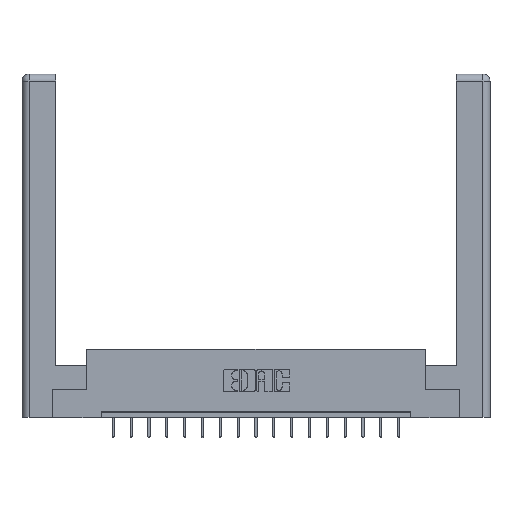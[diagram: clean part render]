
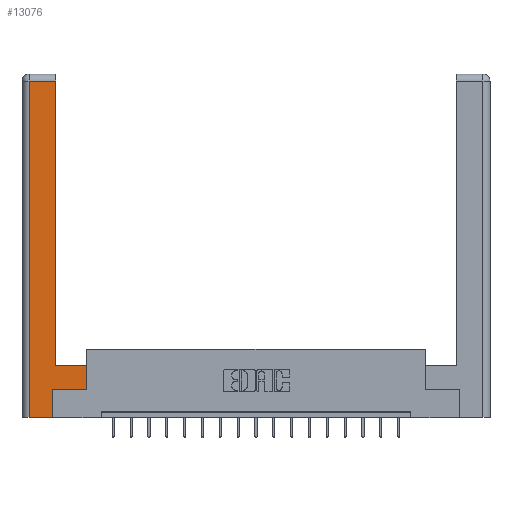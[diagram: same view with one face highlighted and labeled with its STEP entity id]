
A CAD part, top view. The second image highlights one B-rep face of the part: STEP entity #13076.
In plain terms, the highlighted planar face has unit normal (0, 0, 1).
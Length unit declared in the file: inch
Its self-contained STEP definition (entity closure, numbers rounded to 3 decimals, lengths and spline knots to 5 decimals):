
#678 = LINE ( 'NONE', #3868, #5820 ) ;
#895 = VERTEX_POINT ( 'NONE', #13260 ) ;
#1141 = CARTESIAN_POINT ( 'NONE',  ( 0.265, 0.245, 0. ) ) ;
#1548 = VERTEX_POINT ( 'NONE', #1141 ) ;
#2025 = CARTESIAN_POINT ( 'NONE',  ( 0.295, 3., 0. ) ) ;
#2036 = EDGE_CURVE ( 'NONE', #6035, #15443, #678, .T. ) ;
#2357 = DIRECTION ( 'NONE',  ( -1., 0., 0. ) ) ;
#2650 = VECTOR ( 'NONE', #15157, 39.37008 ) ;
#2853 = EDGE_CURVE ( 'NONE', #15443, #895, #17917, .T. ) ;
#3011 = DIRECTION ( 'NONE',  ( 0., 1., 0. ) ) ;
#3128 = DIRECTION ( 'NONE',  ( 1., 0., 0. ) ) ;
#3141 = VECTOR ( 'NONE', #3011, 39.37008 ) ;
#3716 = CARTESIAN_POINT ( 'NONE',  ( 0.265, 0.245, 0. ) ) ;
#3868 = CARTESIAN_POINT ( 'NONE',  ( 0.0615, 2.94, 0. ) ) ;
#4057 = LINE ( 'NONE', #2025, #3141 ) ;
#4668 = ORIENTED_EDGE ( 'NONE', *, *, #13338, .T. ) ;
#5416 = ORIENTED_EDGE ( 'NONE', *, *, #16015, .T. ) ;
#5820 = VECTOR ( 'NONE', #16786, 39.37008 ) ;
#5849 = VERTEX_POINT ( 'NONE', #10890 ) ;
#5963 = CARTESIAN_POINT ( 'NONE',  ( 0.265, 0., 0. ) ) ;
#6035 = VERTEX_POINT ( 'NONE', #12822 ) ;
#6521 = CARTESIAN_POINT ( 'NONE',  ( 0.0615, 0., 0. ) ) ;
#6703 = ORIENTED_EDGE ( 'NONE', *, *, #2036, .T. ) ;
#7491 = EDGE_CURVE ( 'NONE', #5849, #16542, #15803, .T. ) ;
#8021 = CARTESIAN_POINT ( 'NONE',  ( 0.0615, 2.94, 0. ) ) ;
#8182 = CARTESIAN_POINT ( 'NONE',  ( 0.565, 0.245, 0. ) ) ;
#8276 = CARTESIAN_POINT ( 'NONE',  ( 0.295, 0.45, 0. ) ) ;
#8299 = DIRECTION ( 'NONE',  ( 0., 0., -1. ) ) ;
#8716 = EDGE_CURVE ( 'NONE', #15977, #5849, #11734, .T. ) ;
#9403 = ORIENTED_EDGE ( 'NONE', *, *, #10560, .T. ) ;
#9497 = FACE_OUTER_BOUND ( 'NONE', #17702, .T. ) ;
#10161 = LINE ( 'NONE', #8182, #17144 ) ;
#10192 = AXIS2_PLACEMENT_3D ( 'NONE', #16948, #8299, #12683 ) ;
#10560 = EDGE_CURVE ( 'NONE', #16542, #6035, #4057, .T. ) ;
#10890 = CARTESIAN_POINT ( 'NONE',  ( 0.565, 0.45, 0. ) ) ;
#10900 = ORIENTED_EDGE ( 'NONE', *, *, #7491, .T. ) ;
#11194 = CARTESIAN_POINT ( 'NONE',  ( 0.565, 0.245, 0. ) ) ;
#11257 = ORIENTED_EDGE ( 'NONE', *, *, #8716, .T. ) ;
#11321 = VERTEX_POINT ( 'NONE', #15558 ) ;
#11734 = LINE ( 'NONE', #15527, #16218 ) ;
#12008 = VECTOR ( 'NONE', #13823, 39.37008 ) ;
#12489 = LINE ( 'NONE', #3716, #12008 ) ;
#12631 = ORIENTED_EDGE ( 'NONE', *, *, #2853, .T. ) ;
#12665 = VECTOR ( 'NONE', #2357, 39.37008 ) ;
#12683 = DIRECTION ( 'NONE',  ( -1., 0., 0. ) ) ;
#12684 = DIRECTION ( 'NONE',  ( 1., 0., 0. ) ) ;
#12730 = LINE ( 'NONE', #5963, #13642 ) ;
#12822 = CARTESIAN_POINT ( 'NONE',  ( 0.295, 2.94, 0. ) ) ;
#13076 = ADVANCED_FACE ( 'NONE', ( #9497 ), #16886, .F. ) ;
#13260 = CARTESIAN_POINT ( 'NONE',  ( 0.0615, 0., 0. ) ) ;
#13338 = EDGE_CURVE ( 'NONE', #895, #11321, #12730, .T. ) ;
#13642 = VECTOR ( 'NONE', #3128, 39.37008 ) ;
#13823 = DIRECTION ( 'NONE',  ( 0., 1., 0. ) ) ;
#15003 = EDGE_CURVE ( 'NONE', #11321, #1548, #12489, .T. ) ;
#15157 = DIRECTION ( 'NONE',  ( 0., -1., 0. ) ) ;
#15380 = CARTESIAN_POINT ( 'NONE',  ( 0.295, 0.45, 0. ) ) ;
#15443 = VERTEX_POINT ( 'NONE', #8021 ) ;
#15527 = CARTESIAN_POINT ( 'NONE',  ( 0.565, 0.45, 0. ) ) ;
#15558 = CARTESIAN_POINT ( 'NONE',  ( 0.265, 0., 0. ) ) ;
#15803 = LINE ( 'NONE', #15380, #12665 ) ;
#15977 = VERTEX_POINT ( 'NONE', #11194 ) ;
#16015 = EDGE_CURVE ( 'NONE', #1548, #15977, #10161, .T. ) ;
#16218 = VECTOR ( 'NONE', #18499, 39.37008 ) ;
#16542 = VERTEX_POINT ( 'NONE', #8276 ) ;
#16786 = DIRECTION ( 'NONE',  ( -1., 0., 0. ) ) ;
#16886 = PLANE ( 'NONE',  #10192 ) ;
#16948 = CARTESIAN_POINT ( 'NONE',  ( 0., 0., 0. ) ) ;
#17144 = VECTOR ( 'NONE', #12684, 39.37008 ) ;
#17268 = ORIENTED_EDGE ( 'NONE', *, *, #15003, .T. ) ;
#17702 = EDGE_LOOP ( 'NONE', ( #9403, #6703, #12631, #4668, #17268, #5416, #11257, #10900 ) ) ;
#17917 = LINE ( 'NONE', #6521, #2650 ) ;
#18499 = DIRECTION ( 'NONE',  ( 0., 1., 0. ) ) ;
